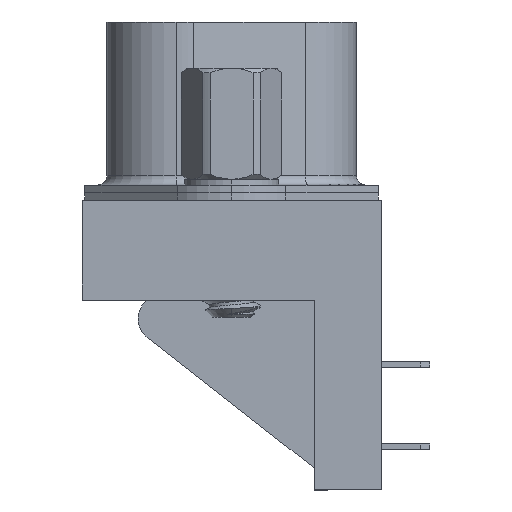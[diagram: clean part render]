
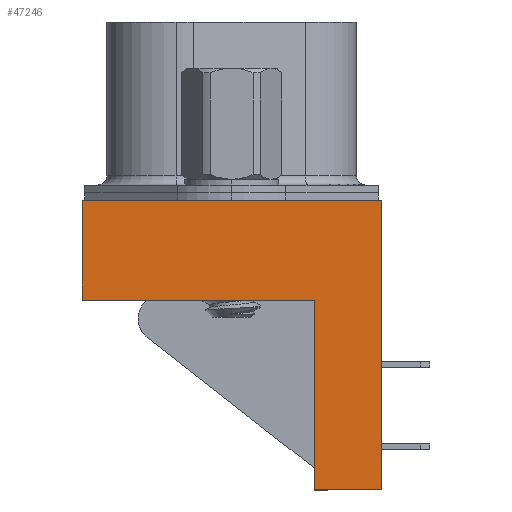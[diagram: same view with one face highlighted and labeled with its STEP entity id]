
A CAD part, left-side view. The second image highlights one B-rep face of the part: STEP entity #47246.
In plain terms, the highlighted planar face has unit normal (-1, 0, 0).
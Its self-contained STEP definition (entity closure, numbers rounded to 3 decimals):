
#6992 = VECTOR ( 'NONE', #83280, 1000. ) ;
#13209 = CARTESIAN_POINT ( 'NONE',  ( -4.125, 7.8, -5.2 ) ) ;
#15356 = CARTESIAN_POINT ( 'NONE',  ( -4.125, 7.8, -15.1 ) ) ;
#22121 = VERTEX_POINT ( 'NONE', #129074 ) ;
#25362 = LINE ( 'NONE', #13209, #6992 ) ;
#31191 = DIRECTION ( 'NONE',  ( 0., -1., 0. ) ) ;
#34040 = LINE ( 'NONE', #90088, #168244 ) ;
#36726 = DIRECTION ( 'NONE',  ( 0., 0., 1. ) ) ;
#41520 = CARTESIAN_POINT ( 'NONE',  ( -4.125, -7.8, -15.1 ) ) ;
#44320 = ORIENTED_EDGE ( 'NONE', *, *, #170214, .F. ) ;
#45344 = EDGE_CURVE ( 'NONE', #63388, #96230, #140474, .T. ) ;
#47246 = ADVANCED_FACE ( 'NONE', ( #56244 ), #127230, .T. ) ;
#48968 = CARTESIAN_POINT ( 'NONE',  ( -4.125, -4.3, -5.2 ) ) ;
#50486 = CARTESIAN_POINT ( 'NONE',  ( -4.125, -7.8, -15.1 ) ) ;
#56244 = FACE_OUTER_BOUND ( 'NONE', #145887, .T. ) ;
#63388 = VERTEX_POINT ( 'NONE', #50486 ) ;
#64937 = VECTOR ( 'NONE', #31191, 1000. ) ;
#69213 = CARTESIAN_POINT ( 'NONE',  ( -4.125, 7.8, -5.2 ) ) ;
#72093 = EDGE_CURVE ( 'NONE', #156167, #63388, #118067, .T. ) ;
#73097 = VECTOR ( 'NONE', #150466, 1000. ) ;
#74350 = EDGE_CURVE ( 'NONE', #22121, #96230, #34040, .T. ) ;
#74868 = VECTOR ( 'NONE', #153549, 1000. ) ;
#78347 = ORIENTED_EDGE ( 'NONE', *, *, #74350, .F. ) ;
#81427 = ORIENTED_EDGE ( 'NONE', *, *, #45344, .T. ) ;
#83280 = DIRECTION ( 'NONE',  ( 0., 1., 0. ) ) ;
#90088 = CARTESIAN_POINT ( 'NONE',  ( -4.125, 7.8, 0. ) ) ;
#96230 = VERTEX_POINT ( 'NONE', #177249 ) ;
#97654 = VECTOR ( 'NONE', #36726, 1000. ) ;
#101969 = DIRECTION ( 'NONE',  ( 0., -1., 0. ) ) ;
#102881 = CARTESIAN_POINT ( 'NONE',  ( -4.125, 7.8, -15.1 ) ) ;
#118067 = LINE ( 'NONE', #15356, #64937 ) ;
#119865 = CARTESIAN_POINT ( 'NONE',  ( -4.125, 7.8, -15.1 ) ) ;
#126095 = EDGE_CURVE ( 'NONE', #156167, #136992, #166325, .T. ) ;
#127230 = PLANE ( 'NONE',  #135161 ) ;
#129074 = CARTESIAN_POINT ( 'NONE',  ( -4.125, 7.8, 0. ) ) ;
#130091 = EDGE_CURVE ( 'NONE', #184514, #22121, #150607, .T. ) ;
#135161 = AXIS2_PLACEMENT_3D ( 'NONE', #102881, #144852, #101969 ) ;
#136992 = VERTEX_POINT ( 'NONE', #48968 ) ;
#139683 = ORIENTED_EDGE ( 'NONE', *, *, #72093, .T. ) ;
#140474 = LINE ( 'NONE', #41520, #74868 ) ;
#144852 = DIRECTION ( 'NONE',  ( -1., 0., 0. ) ) ;
#145887 = EDGE_LOOP ( 'NONE', ( #44320, #159855, #139683, #81427, #78347, #171167 ) ) ;
#150466 = DIRECTION ( 'NONE',  ( 0., 0., 1. ) ) ;
#150607 = LINE ( 'NONE', #119865, #97654 ) ;
#153549 = DIRECTION ( 'NONE',  ( 0., 0., 1. ) ) ;
#156167 = VERTEX_POINT ( 'NONE', #181129 ) ;
#159855 = ORIENTED_EDGE ( 'NONE', *, *, #126095, .F. ) ;
#166325 = LINE ( 'NONE', #167246, #73097 ) ;
#167246 = CARTESIAN_POINT ( 'NONE',  ( -4.125, -4.3, -15.1 ) ) ;
#168244 = VECTOR ( 'NONE', #173179, 1000. ) ;
#170214 = EDGE_CURVE ( 'NONE', #136992, #184514, #25362, .T. ) ;
#171167 = ORIENTED_EDGE ( 'NONE', *, *, #130091, .F. ) ;
#173179 = DIRECTION ( 'NONE',  ( 0., -1., 0. ) ) ;
#177249 = CARTESIAN_POINT ( 'NONE',  ( -4.125, -7.8, 0. ) ) ;
#181129 = CARTESIAN_POINT ( 'NONE',  ( -4.125, -4.3, -15.1 ) ) ;
#184514 = VERTEX_POINT ( 'NONE', #69213 ) ;
